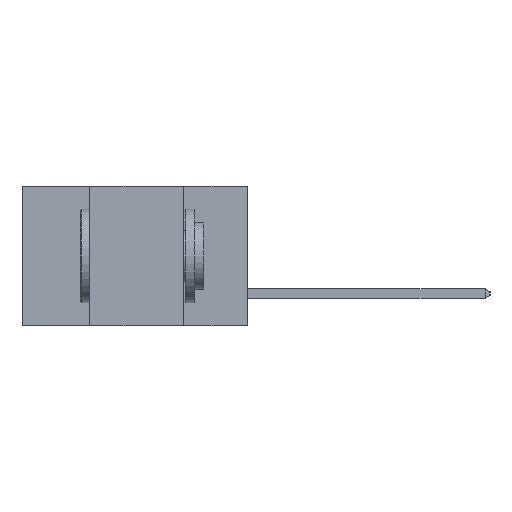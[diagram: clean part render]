
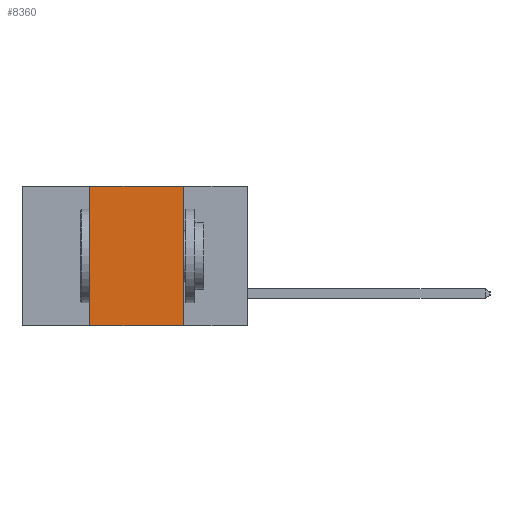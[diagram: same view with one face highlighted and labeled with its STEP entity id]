
A CAD part, left-side view. The second image highlights one B-rep face of the part: STEP entity #8360.
In plain terms, the highlighted planar face has unit normal (-1, 0, 0).
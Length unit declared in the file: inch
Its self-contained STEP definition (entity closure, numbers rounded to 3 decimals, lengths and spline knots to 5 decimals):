
#315 = CARTESIAN_POINT ( 'NONE',  ( 0., 0.17, 0. ) ) ;
#340 = VERTEX_POINT ( 'NONE', #9366 ) ;
#510 = AXIS2_PLACEMENT_3D ( 'NONE', #10062, #8164, #2023 ) ;
#550 = FACE_OUTER_BOUND ( 'NONE', #932, .T. ) ;
#575 = VECTOR ( 'NONE', #2511, 39.37008 ) ;
#810 = VERTEX_POINT ( 'NONE', #1830 ) ;
#932 = EDGE_LOOP ( 'NONE', ( #7113, #1944, #2619, #5406 ) ) ;
#951 = PLANE ( 'NONE',  #510 ) ;
#1145 = EDGE_CURVE ( 'NONE', #810, #1350, #3900, .T. ) ;
#1261 = VERTEX_POINT ( 'NONE', #6105 ) ;
#1350 = VERTEX_POINT ( 'NONE', #315 ) ;
#1830 = CARTESIAN_POINT ( 'NONE',  ( 0., 0.42, 0. ) ) ;
#1944 = ORIENTED_EDGE ( 'NONE', *, *, #1145, .F. ) ;
#2023 = DIRECTION ( 'NONE',  ( 0., 0., -1. ) ) ;
#2511 = DIRECTION ( 'NONE',  ( 0., 0., -1. ) ) ;
#2619 = ORIENTED_EDGE ( 'NONE', *, *, #6796, .F. ) ;
#3160 = LINE ( 'NONE', #7972, #10817 ) ;
#3403 = EDGE_CURVE ( 'NONE', #1261, #340, #3160, .T. ) ;
#3431 = LINE ( 'NONE', #4585, #575 ) ;
#3614 = VECTOR ( 'NONE', #7579, 39.37008 ) ;
#3900 = LINE ( 'NONE', #10667, #11791 ) ;
#4585 = CARTESIAN_POINT ( 'NONE',  ( 0., 0.17, 0. ) ) ;
#5406 = ORIENTED_EDGE ( 'NONE', *, *, #3403, .T. ) ;
#6105 = CARTESIAN_POINT ( 'NONE',  ( 0., 0.42, -0.37 ) ) ;
#6796 = EDGE_CURVE ( 'NONE', #1261, #810, #9257, .T. ) ;
#7113 = ORIENTED_EDGE ( 'NONE', *, *, #7461, .F. ) ;
#7461 = EDGE_CURVE ( 'NONE', #1350, #340, #3431, .T. ) ;
#7579 = DIRECTION ( 'NONE',  ( 0., 0., 1. ) ) ;
#7972 = CARTESIAN_POINT ( 'NONE',  ( 0., 0.6, -0.37 ) ) ;
#8164 = DIRECTION ( 'NONE',  ( 1., 0., 0. ) ) ;
#8360 = ADVANCED_FACE ( 'NONE', ( #550 ), #951, .F. ) ;
#9257 = LINE ( 'NONE', #9576, #3614 ) ;
#9366 = CARTESIAN_POINT ( 'NONE',  ( 0., 0.17, -0.37 ) ) ;
#9576 = CARTESIAN_POINT ( 'NONE',  ( 0., 0.42, 0. ) ) ;
#10062 = CARTESIAN_POINT ( 'NONE',  ( 0., 0.6, 0. ) ) ;
#10667 = CARTESIAN_POINT ( 'NONE',  ( 0., 0.6, 0. ) ) ;
#10679 = DIRECTION ( 'NONE',  ( 0., -1., 0. ) ) ;
#10817 = VECTOR ( 'NONE', #10847, 39.37008 ) ;
#10847 = DIRECTION ( 'NONE',  ( 0., -1., 0. ) ) ;
#11791 = VECTOR ( 'NONE', #10679, 39.37008 ) ;
